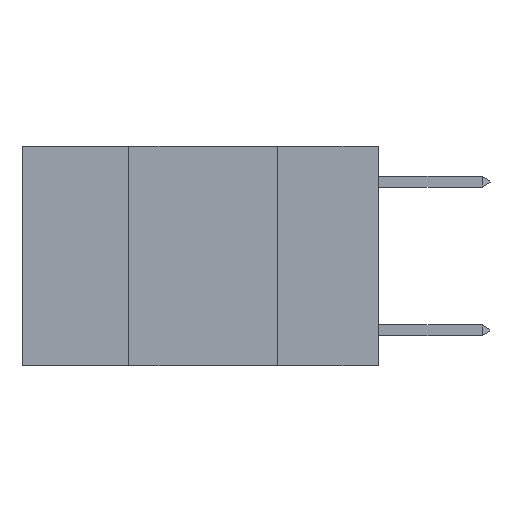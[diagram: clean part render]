
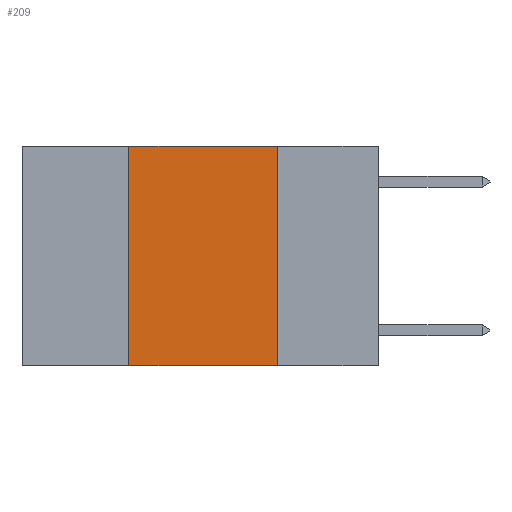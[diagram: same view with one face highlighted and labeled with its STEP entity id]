
A CAD part, left-side view. The second image highlights one B-rep face of the part: STEP entity #209.
In plain terms, the highlighted planar face has unit normal (-1, 0, 0).
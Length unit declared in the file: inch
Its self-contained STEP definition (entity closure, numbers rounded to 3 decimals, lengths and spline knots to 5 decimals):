
#148 = DIRECTION ( 'NONE',  ( 1., 0., 0. ) ) ;
#209 = ADVANCED_FACE ( 'NONE', ( #2272 ), #5692, .F. ) ;
#267 = ORIENTED_EDGE ( 'NONE', *, *, #1439, .F. ) ;
#349 = CARTESIAN_POINT ( 'NONE',  ( 0., 0.42, 0. ) ) ;
#941 = LINE ( 'NONE', #7172, #2070 ) ;
#1071 = CARTESIAN_POINT ( 'NONE',  ( 0., 0.17, -0.37 ) ) ;
#1288 = VERTEX_POINT ( 'NONE', #349 ) ;
#1439 = EDGE_CURVE ( 'NONE', #2841, #1288, #7478, .T. ) ;
#1681 = DIRECTION ( 'NONE',  ( 0., 0., -1. ) ) ;
#2070 = VECTOR ( 'NONE', #1681, 39.37008 ) ;
#2072 = VECTOR ( 'NONE', #4142, 39.37008 ) ;
#2078 = VECTOR ( 'NONE', #4154, 39.37008 ) ;
#2091 = EDGE_LOOP ( 'NONE', ( #7974, #7102, #267, #3156 ) ) ;
#2272 = FACE_OUTER_BOUND ( 'NONE', #2091, .T. ) ;
#2394 = AXIS2_PLACEMENT_3D ( 'NONE', #2945, #148, #4819 ) ;
#2412 = EDGE_CURVE ( 'NONE', #1288, #8392, #8818, .T. ) ;
#2841 = VERTEX_POINT ( 'NONE', #6067 ) ;
#2945 = CARTESIAN_POINT ( 'NONE',  ( 0., 0.6, 0. ) ) ;
#3156 = ORIENTED_EDGE ( 'NONE', *, *, #6145, .T. ) ;
#4142 = DIRECTION ( 'NONE',  ( 0., 0., 1. ) ) ;
#4154 = DIRECTION ( 'NONE',  ( 0., -1., 0. ) ) ;
#4505 = CARTESIAN_POINT ( 'NONE',  ( 0., 0.17, 0. ) ) ;
#4819 = DIRECTION ( 'NONE',  ( 0., 0., -1. ) ) ;
#4820 = CARTESIAN_POINT ( 'NONE',  ( 0., 0.42, 0. ) ) ;
#5692 = PLANE ( 'NONE',  #2394 ) ;
#5897 = VECTOR ( 'NONE', #8326, 39.37008 ) ;
#6013 = VERTEX_POINT ( 'NONE', #1071 ) ;
#6067 = CARTESIAN_POINT ( 'NONE',  ( 0., 0.42, -0.37 ) ) ;
#6093 = LINE ( 'NONE', #7648, #5897 ) ;
#6145 = EDGE_CURVE ( 'NONE', #2841, #6013, #6093, .T. ) ;
#7102 = ORIENTED_EDGE ( 'NONE', *, *, #2412, .F. ) ;
#7172 = CARTESIAN_POINT ( 'NONE',  ( 0., 0.17, 0. ) ) ;
#7478 = LINE ( 'NONE', #4820, #2072 ) ;
#7589 = CARTESIAN_POINT ( 'NONE',  ( 0., 0.6, 0. ) ) ;
#7648 = CARTESIAN_POINT ( 'NONE',  ( 0., 0.6, -0.37 ) ) ;
#7974 = ORIENTED_EDGE ( 'NONE', *, *, #8282, .F. ) ;
#8282 = EDGE_CURVE ( 'NONE', #8392, #6013, #941, .T. ) ;
#8326 = DIRECTION ( 'NONE',  ( 0., -1., 0. ) ) ;
#8392 = VERTEX_POINT ( 'NONE', #4505 ) ;
#8818 = LINE ( 'NONE', #7589, #2078 ) ;
